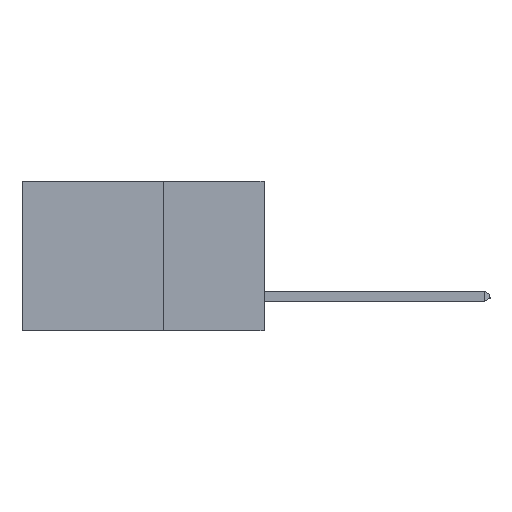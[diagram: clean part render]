
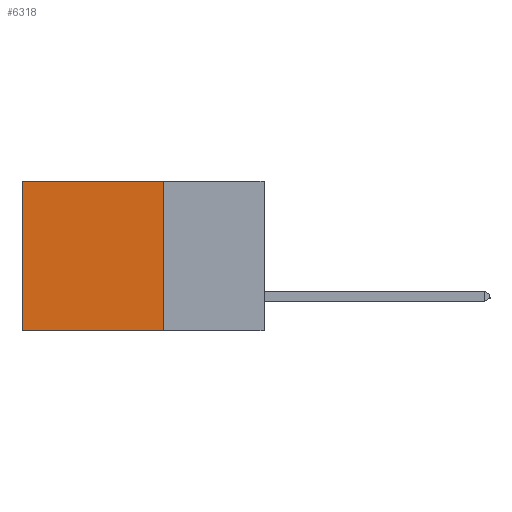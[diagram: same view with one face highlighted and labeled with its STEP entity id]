
A CAD part, left-side view. The second image highlights one B-rep face of the part: STEP entity #6318.
In plain terms, the highlighted planar face has unit normal (-1, 0, 0).
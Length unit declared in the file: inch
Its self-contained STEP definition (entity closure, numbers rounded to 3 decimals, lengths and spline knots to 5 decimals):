
#96 = VECTOR ( 'NONE', #13885, 39.37008 ) ;
#120 = DIRECTION ( 'NONE',  ( 0., 1., 0. ) ) ;
#660 = CARTESIAN_POINT ( 'NONE',  ( 0.298, 0.6, 0. ) ) ;
#670 = AXIS2_PLACEMENT_3D ( 'NONE', #12342, #12322, #12235 ) ;
#750 = DIRECTION ( 'NONE',  ( 0., 0., -1. ) ) ;
#1143 = DIRECTION ( 'NONE',  ( 0., 1., 0. ) ) ;
#1243 = CARTESIAN_POINT ( 'NONE',  ( 0.298, 0.25, -0.37 ) ) ;
#2915 = EDGE_CURVE ( 'NONE', #4530, #7758, #10864, .T. ) ;
#3119 = CARTESIAN_POINT ( 'NONE',  ( 0.298, 0.6, -0.37 ) ) ;
#3949 = VERTEX_POINT ( 'NONE', #1243 ) ;
#4515 = CARTESIAN_POINT ( 'NONE',  ( 0.298, 0.25, 0. ) ) ;
#4530 = VERTEX_POINT ( 'NONE', #6536 ) ;
#4661 = CARTESIAN_POINT ( 'NONE',  ( 0.298, 0.25, 0. ) ) ;
#5528 = EDGE_CURVE ( 'NONE', #7758, #15095, #8794, .T. ) ;
#5731 = VECTOR ( 'NONE', #1143, 39.37008 ) ;
#5907 = EDGE_LOOP ( 'NONE', ( #12757, #12068, #8864, #12033 ) ) ;
#6318 = ADVANCED_FACE ( 'NONE', ( #6344 ), #12734, .F. ) ;
#6344 = FACE_OUTER_BOUND ( 'NONE', #5907, .T. ) ;
#6536 = CARTESIAN_POINT ( 'NONE',  ( 0.298, 0.25, 0. ) ) ;
#6891 = LINE ( 'NONE', #4515, #96 ) ;
#7410 = VECTOR ( 'NONE', #120, 39.37008 ) ;
#7758 = VERTEX_POINT ( 'NONE', #11021 ) ;
#8794 = LINE ( 'NONE', #660, #11474 ) ;
#8864 = ORIENTED_EDGE ( 'NONE', *, *, #12877, .F. ) ;
#10864 = LINE ( 'NONE', #4661, #7410 ) ;
#11021 = CARTESIAN_POINT ( 'NONE',  ( 0.298, 0.6, 0. ) ) ;
#11474 = VECTOR ( 'NONE', #750, 39.37008 ) ;
#11929 = LINE ( 'NONE', #15202, #5731 ) ;
#12033 = ORIENTED_EDGE ( 'NONE', *, *, #2915, .T. ) ;
#12068 = ORIENTED_EDGE ( 'NONE', *, *, #14547, .F. ) ;
#12235 = DIRECTION ( 'NONE',  ( 0., 0., -1. ) ) ;
#12322 = DIRECTION ( 'NONE',  ( 1., 0., 0. ) ) ;
#12342 = CARTESIAN_POINT ( 'NONE',  ( 0.298, 0.25, 0. ) ) ;
#12734 = PLANE ( 'NONE',  #670 ) ;
#12757 = ORIENTED_EDGE ( 'NONE', *, *, #5528, .T. ) ;
#12877 = EDGE_CURVE ( 'NONE', #4530, #3949, #6891, .T. ) ;
#13885 = DIRECTION ( 'NONE',  ( 0., 0., -1. ) ) ;
#14547 = EDGE_CURVE ( 'NONE', #3949, #15095, #11929, .T. ) ;
#15095 = VERTEX_POINT ( 'NONE', #3119 ) ;
#15202 = CARTESIAN_POINT ( 'NONE',  ( 0.298, 0.25, -0.37 ) ) ;
